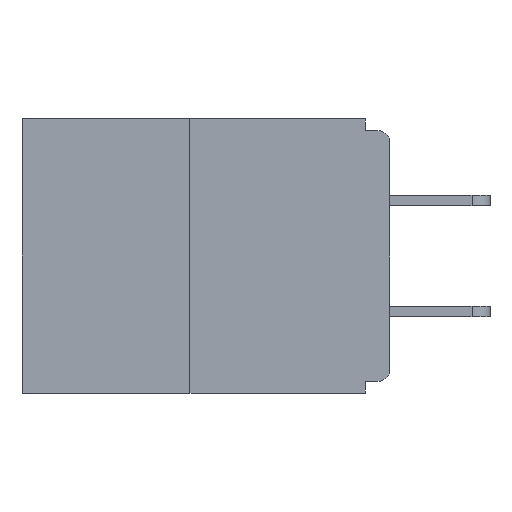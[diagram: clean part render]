
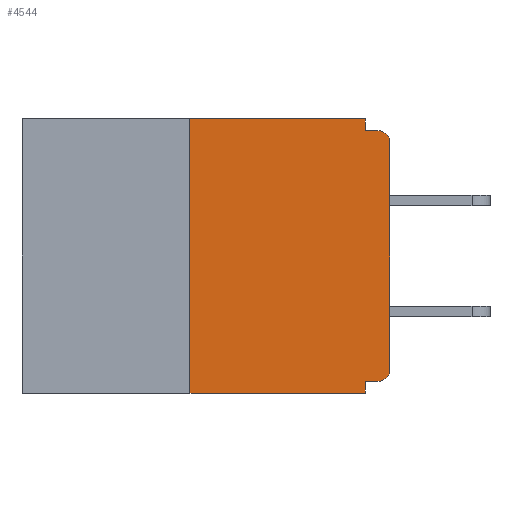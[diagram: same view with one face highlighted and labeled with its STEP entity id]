
A CAD part, left-side view. The second image highlights one B-rep face of the part: STEP entity #4544.
In plain terms, the highlighted planar face has unit normal (-1, 0, 0).
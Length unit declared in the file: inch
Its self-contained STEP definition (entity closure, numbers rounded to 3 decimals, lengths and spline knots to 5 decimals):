
#133 = CARTESIAN_POINT ( 'NONE',  ( 0., 0.25, -0.343 ) ) ;
#395 = LINE ( 'NONE', #10765, #1918 ) ;
#854 = DIRECTION ( 'NONE',  ( 0., -1., 0. ) ) ;
#900 = DIRECTION ( 'NONE',  ( 0., 0., -1. ) ) ;
#905 = LINE ( 'NONE', #11791, #1249 ) ;
#955 = DIRECTION ( 'NONE',  ( 0., 0., 1. ) ) ;
#1249 = VECTOR ( 'NONE', #854, 39.37008 ) ;
#1699 = EDGE_CURVE ( 'NONE', #12448, #12114, #395, .T. ) ;
#1789 = DIRECTION ( 'NONE',  ( -1., 0., 0. ) ) ;
#1893 = CARTESIAN_POINT ( 'NONE',  ( 0., 0.015, -0.015 ) ) ;
#1918 = VECTOR ( 'NONE', #3522, 39.37008 ) ;
#2296 = VERTEX_POINT ( 'NONE', #8528 ) ;
#2366 = FACE_OUTER_BOUND ( 'NONE', #9302, .T. ) ;
#2997 = CIRCLE ( 'NONE', #9139, 0.015 ) ;
#3017 = EDGE_CURVE ( 'NONE', #7382, #7776, #905, .T. ) ;
#3027 = CARTESIAN_POINT ( 'NONE',  ( 0., 0.25, 0. ) ) ;
#3052 = EDGE_CURVE ( 'NONE', #12114, #7382, #12805, .T. ) ;
#3083 = ORIENTED_EDGE ( 'NONE', *, *, #3017, .F. ) ;
#3154 = CARTESIAN_POINT ( 'NONE',  ( 0., 0.031, 0. ) ) ;
#3208 = DIRECTION ( 'NONE',  ( 0., 1., 0. ) ) ;
#3354 = LINE ( 'NONE', #5690, #9433 ) ;
#3482 = DIRECTION ( 'NONE',  ( 0., -1., 0. ) ) ;
#3522 = DIRECTION ( 'NONE',  ( 0., -1., 0. ) ) ;
#3696 = EDGE_CURVE ( 'NONE', #6662, #2296, #8299, .T. ) ;
#3758 = VERTEX_POINT ( 'NONE', #133 ) ;
#3792 = DIRECTION ( 'NONE',  ( -1., 0., 0. ) ) ;
#3929 = DIRECTION ( 'NONE',  ( 0., 0., -1. ) ) ;
#4089 = ORIENTED_EDGE ( 'NONE', *, *, #11361, .F. ) ;
#4324 = VECTOR ( 'NONE', #955, 39.37008 ) ;
#4544 = ADVANCED_FACE ( 'NONE', ( #2366 ), #5465, .F. ) ;
#4656 = CARTESIAN_POINT ( 'NONE',  ( 0., 0.46, -0.343 ) ) ;
#4815 = CARTESIAN_POINT ( 'NONE',  ( 0., 0.031, -0.343 ) ) ;
#5465 = PLANE ( 'NONE',  #10469 ) ;
#5466 = ORIENTED_EDGE ( 'NONE', *, *, #10142, .T. ) ;
#5690 = CARTESIAN_POINT ( 'NONE',  ( 0., 0., 0. ) ) ;
#5894 = CARTESIAN_POINT ( 'NONE',  ( 0., 0.015, -0.03 ) ) ;
#6019 = CARTESIAN_POINT ( 'NONE',  ( 0., 0.015, -0.328 ) ) ;
#6326 = EDGE_CURVE ( 'NONE', #6662, #11793, #2997, .T. ) ;
#6376 = ORIENTED_EDGE ( 'NONE', *, *, #1699, .F. ) ;
#6495 = LINE ( 'NONE', #11376, #10230 ) ;
#6539 = DIRECTION ( 'NONE',  ( 1., 0., 0. ) ) ;
#6662 = VERTEX_POINT ( 'NONE', #6019 ) ;
#6699 = ORIENTED_EDGE ( 'NONE', *, *, #3696, .F. ) ;
#6733 = EDGE_CURVE ( 'NONE', #3758, #12448, #7178, .T. ) ;
#6773 = VECTOR ( 'NONE', #3482, 39.37008 ) ;
#7178 = LINE ( 'NONE', #3027, #4324 ) ;
#7382 = VERTEX_POINT ( 'NONE', #10760 ) ;
#7498 = VERTEX_POINT ( 'NONE', #7749 ) ;
#7585 = ORIENTED_EDGE ( 'NONE', *, *, #8459, .T. ) ;
#7734 = ORIENTED_EDGE ( 'NONE', *, *, #9965, .T. ) ;
#7749 = CARTESIAN_POINT ( 'NONE',  ( 0., 0., -0.03 ) ) ;
#7776 = VERTEX_POINT ( 'NONE', #1893 ) ;
#8242 = ORIENTED_EDGE ( 'NONE', *, *, #6326, .T. ) ;
#8299 = LINE ( 'NONE', #8613, #9480 ) ;
#8362 = CARTESIAN_POINT ( 'NONE',  ( 0., 0., -0.313 ) ) ;
#8459 = EDGE_CURVE ( 'NONE', #3758, #13557, #12811, .T. ) ;
#8528 = CARTESIAN_POINT ( 'NONE',  ( 0., 0.031, -0.328 ) ) ;
#8568 = CIRCLE ( 'NONE', #9444, 0.015 ) ;
#8613 = CARTESIAN_POINT ( 'NONE',  ( 0., 0., -0.328 ) ) ;
#9139 = AXIS2_PLACEMENT_3D ( 'NONE', #13560, #1789, #11523 ) ;
#9219 = CARTESIAN_POINT ( 'NONE',  ( 0., 0.031, 0. ) ) ;
#9302 = EDGE_LOOP ( 'NONE', ( #6376, #9986, #7585, #4089, #6699, #8242, #5466, #7734, #3083, #11115 ) ) ;
#9433 = VECTOR ( 'NONE', #12235, 39.37008 ) ;
#9444 = AXIS2_PLACEMENT_3D ( 'NONE', #5894, #3792, #3929 ) ;
#9480 = VECTOR ( 'NONE', #3208, 39.37008 ) ;
#9860 = DIRECTION ( 'NONE',  ( 0., 0., -1. ) ) ;
#9965 = EDGE_CURVE ( 'NONE', #7498, #7776, #8568, .T. ) ;
#9986 = ORIENTED_EDGE ( 'NONE', *, *, #6733, .F. ) ;
#10004 = VECTOR ( 'NONE', #900, 39.37008 ) ;
#10142 = EDGE_CURVE ( 'NONE', #11793, #7498, #3354, .T. ) ;
#10230 = VECTOR ( 'NONE', #11242, 39.37008 ) ;
#10469 = AXIS2_PLACEMENT_3D ( 'NONE', #10898, #6539, #9860 ) ;
#10760 = CARTESIAN_POINT ( 'NONE',  ( 0., 0.031, -0.015 ) ) ;
#10765 = CARTESIAN_POINT ( 'NONE',  ( 0., 0.46, 0. ) ) ;
#10898 = CARTESIAN_POINT ( 'NONE',  ( 0., 0.46, 0. ) ) ;
#11115 = ORIENTED_EDGE ( 'NONE', *, *, #3052, .F. ) ;
#11242 = DIRECTION ( 'NONE',  ( 0., 0., -1. ) ) ;
#11282 = CARTESIAN_POINT ( 'NONE',  ( 0., 0.25, 0. ) ) ;
#11361 = EDGE_CURVE ( 'NONE', #2296, #13557, #6495, .T. ) ;
#11376 = CARTESIAN_POINT ( 'NONE',  ( 0., 0.031, -0.343 ) ) ;
#11523 = DIRECTION ( 'NONE',  ( 0., 0., -1. ) ) ;
#11791 = CARTESIAN_POINT ( 'NONE',  ( 0., 0., -0.015 ) ) ;
#11793 = VERTEX_POINT ( 'NONE', #8362 ) ;
#12114 = VERTEX_POINT ( 'NONE', #9219 ) ;
#12235 = DIRECTION ( 'NONE',  ( 0., 0., 1. ) ) ;
#12448 = VERTEX_POINT ( 'NONE', #11282 ) ;
#12805 = LINE ( 'NONE', #3154, #10004 ) ;
#12811 = LINE ( 'NONE', #4656, #6773 ) ;
#13557 = VERTEX_POINT ( 'NONE', #4815 ) ;
#13560 = CARTESIAN_POINT ( 'NONE',  ( 0., 0.015, -0.313 ) ) ;
